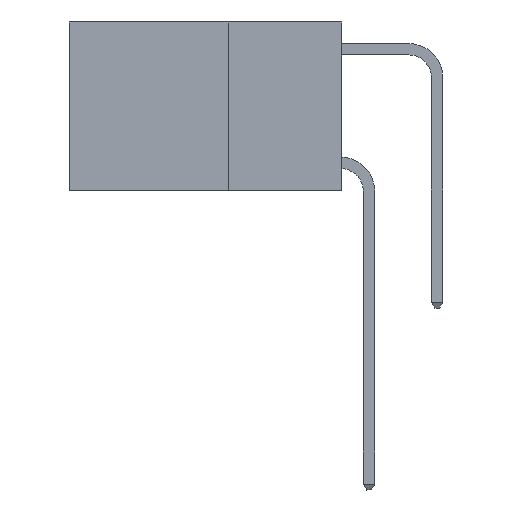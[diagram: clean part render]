
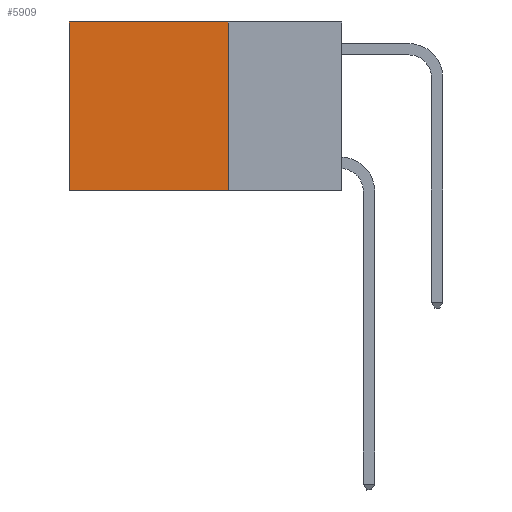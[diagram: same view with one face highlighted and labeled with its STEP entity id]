
A CAD part, left-side view. The second image highlights one B-rep face of the part: STEP entity #5909.
In plain terms, the highlighted planar face has unit normal (-1, 0, 0).
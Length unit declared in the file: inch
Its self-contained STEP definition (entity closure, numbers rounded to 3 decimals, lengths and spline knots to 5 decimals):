
#173 = ORIENTED_EDGE ( 'NONE', *, *, #5916, .T. ) ;
#271 = LINE ( 'NONE', #6755, #3721 ) ;
#351 = CARTESIAN_POINT ( 'NONE',  ( 0.2625, 0.6, 0. ) ) ;
#421 = VECTOR ( 'NONE', #11996, 39.37008 ) ;
#457 = CARTESIAN_POINT ( 'NONE',  ( 0.2625, 0.25, -0.37 ) ) ;
#651 = VERTEX_POINT ( 'NONE', #6874 ) ;
#657 = EDGE_CURVE ( 'NONE', #12775, #8399, #9215, .T. ) ;
#764 = ORIENTED_EDGE ( 'NONE', *, *, #4317, .F. ) ;
#1709 = VECTOR ( 'NONE', #6636, 39.37008 ) ;
#2886 = VERTEX_POINT ( 'NONE', #457 ) ;
#3721 = VECTOR ( 'NONE', #14562, 39.37008 ) ;
#4317 = EDGE_CURVE ( 'NONE', #2886, #8399, #12147, .T. ) ;
#4430 = DIRECTION ( 'NONE',  ( 0., 0., -1. ) ) ;
#5234 = CARTESIAN_POINT ( 'NONE',  ( 0.2625, 0.6, 0. ) ) ;
#5909 = ADVANCED_FACE ( 'NONE', ( #6444 ), #10078, .F. ) ;
#5916 = EDGE_CURVE ( 'NONE', #651, #12775, #271, .T. ) ;
#6444 = FACE_OUTER_BOUND ( 'NONE', #9145, .T. ) ;
#6636 = DIRECTION ( 'NONE',  ( 0., 0., -1. ) ) ;
#6647 = AXIS2_PLACEMENT_3D ( 'NONE', #6696, #11256, #4430 ) ;
#6696 = CARTESIAN_POINT ( 'NONE',  ( 0.2625, 0.25, 0. ) ) ;
#6755 = CARTESIAN_POINT ( 'NONE',  ( 0.2625, 0.25, 0. ) ) ;
#6874 = CARTESIAN_POINT ( 'NONE',  ( 0.2625, 0.25, 0. ) ) ;
#7815 = LINE ( 'NONE', #8854, #1709 ) ;
#8090 = EDGE_CURVE ( 'NONE', #651, #2886, #7815, .T. ) ;
#8399 = VERTEX_POINT ( 'NONE', #13923 ) ;
#8846 = CARTESIAN_POINT ( 'NONE',  ( 0.2625, 0.25, -0.37 ) ) ;
#8854 = CARTESIAN_POINT ( 'NONE',  ( 0.2625, 0.25, 0. ) ) ;
#8994 = ORIENTED_EDGE ( 'NONE', *, *, #657, .T. ) ;
#9145 = EDGE_LOOP ( 'NONE', ( #8994, #764, #9885, #173 ) ) ;
#9215 = LINE ( 'NONE', #351, #421 ) ;
#9885 = ORIENTED_EDGE ( 'NONE', *, *, #8090, .F. ) ;
#9975 = DIRECTION ( 'NONE',  ( 0., 1., 0. ) ) ;
#10078 = PLANE ( 'NONE',  #6647 ) ;
#11256 = DIRECTION ( 'NONE',  ( 1., 0., 0. ) ) ;
#11435 = VECTOR ( 'NONE', #9975, 39.37008 ) ;
#11996 = DIRECTION ( 'NONE',  ( 0., 0., -1. ) ) ;
#12147 = LINE ( 'NONE', #8846, #11435 ) ;
#12775 = VERTEX_POINT ( 'NONE', #5234 ) ;
#13923 = CARTESIAN_POINT ( 'NONE',  ( 0.2625, 0.6, -0.37 ) ) ;
#14562 = DIRECTION ( 'NONE',  ( 0., 1., 0. ) ) ;
